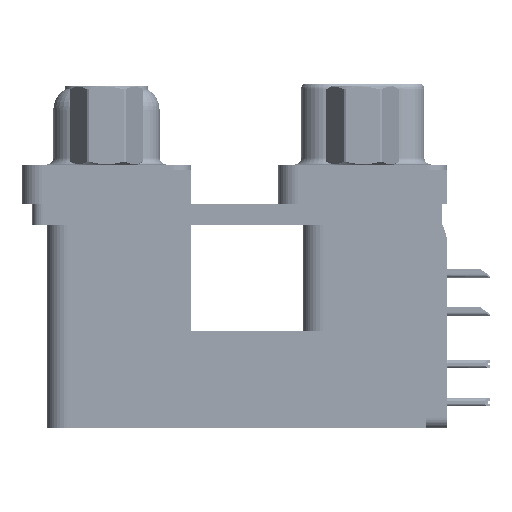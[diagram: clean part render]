
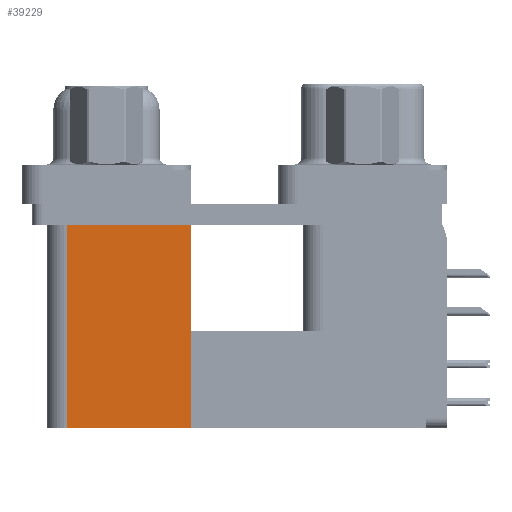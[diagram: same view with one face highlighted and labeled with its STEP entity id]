
A CAD part, left-side view. The second image highlights one B-rep face of the part: STEP entity #39229.
In plain terms, the highlighted planar face has unit normal (-1, 0, 0).
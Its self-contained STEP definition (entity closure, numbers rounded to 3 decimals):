
#2936 = VECTOR ( 'NONE', #23144, 1000. ) ;
#5720 = VECTOR ( 'NONE', #35693, 1000. ) ;
#10803 = VERTEX_POINT ( 'NONE', #59723 ) ;
#11583 = PLANE ( 'NONE',  #20371 ) ;
#13840 = LINE ( 'NONE', #50321, #2936 ) ;
#14772 = EDGE_LOOP ( 'NONE', ( #29791, #48993, #52065, #41909 ) ) ;
#16425 = DIRECTION ( 'NONE',  ( 0., 0., -1. ) ) ;
#18125 = CARTESIAN_POINT ( 'NONE',  ( 3.7, 12.775, -19.2 ) ) ;
#19304 = CARTESIAN_POINT ( 'NONE',  ( 3.7, 21.975, -2.5 ) ) ;
#20135 = CARTESIAN_POINT ( 'NONE',  ( 3.7, 12.775, -19.2 ) ) ;
#20371 = AXIS2_PLACEMENT_3D ( 'NONE', #43276, #57760, #16425 ) ;
#20926 = FACE_OUTER_BOUND ( 'NONE', #14772, .T. ) ;
#23144 = DIRECTION ( 'NONE',  ( 0., 0., 1. ) ) ;
#29791 = ORIENTED_EDGE ( 'NONE', *, *, #54209, .T. ) ;
#31205 = VECTOR ( 'NONE', #41059, 1000. ) ;
#32566 = CARTESIAN_POINT ( 'NONE',  ( 3.7, 12.775, -19.2 ) ) ;
#33556 = VERTEX_POINT ( 'NONE', #19304 ) ;
#35693 = DIRECTION ( 'NONE',  ( 0., 1., 0. ) ) ;
#36234 = LINE ( 'NONE', #18125, #31205 ) ;
#36347 = EDGE_CURVE ( 'NONE', #56059, #10803, #51840, .T. ) ;
#38327 = EDGE_CURVE ( 'NONE', #10803, #33556, #13840, .T. ) ;
#39229 = ADVANCED_FACE ( 'NONE', ( #20926 ), #11583, .F. ) ;
#41059 = DIRECTION ( 'NONE',  ( 0., 0., 1. ) ) ;
#41701 = CARTESIAN_POINT ( 'NONE',  ( 3.7, 12.775, -2.5 ) ) ;
#41909 = ORIENTED_EDGE ( 'NONE', *, *, #49174, .T. ) ;
#43276 = CARTESIAN_POINT ( 'NONE',  ( 3.7, 12.775, -19.2 ) ) ;
#46991 = DIRECTION ( 'NONE',  ( 0., 1., 0. ) ) ;
#48833 = VERTEX_POINT ( 'NONE', #41701 ) ;
#48993 = ORIENTED_EDGE ( 'NONE', *, *, #38327, .F. ) ;
#49174 = EDGE_CURVE ( 'NONE', #56059, #48833, #36234, .T. ) ;
#49560 = LINE ( 'NONE', #58655, #5720 ) ;
#50321 = CARTESIAN_POINT ( 'NONE',  ( 3.7, 21.975, -19.2 ) ) ;
#51840 = LINE ( 'NONE', #20135, #59499 ) ;
#52065 = ORIENTED_EDGE ( 'NONE', *, *, #36347, .F. ) ;
#54209 = EDGE_CURVE ( 'NONE', #48833, #33556, #49560, .T. ) ;
#56059 = VERTEX_POINT ( 'NONE', #32566 ) ;
#57760 = DIRECTION ( 'NONE',  ( 1., 0., 0. ) ) ;
#58655 = CARTESIAN_POINT ( 'NONE',  ( 3.7, 12.775, -2.5 ) ) ;
#59499 = VECTOR ( 'NONE', #46991, 1000. ) ;
#59723 = CARTESIAN_POINT ( 'NONE',  ( 3.7, 21.975, -19.2 ) ) ;
